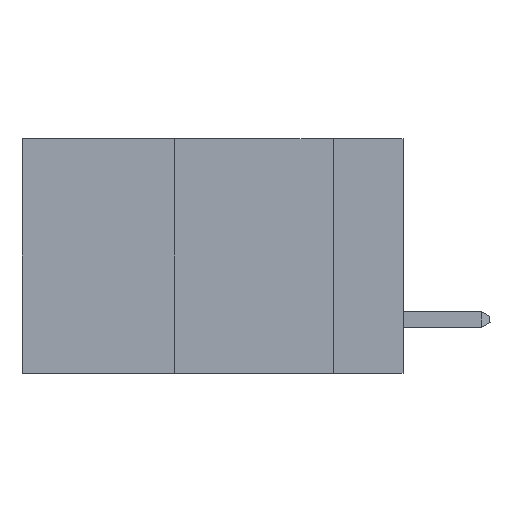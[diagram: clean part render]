
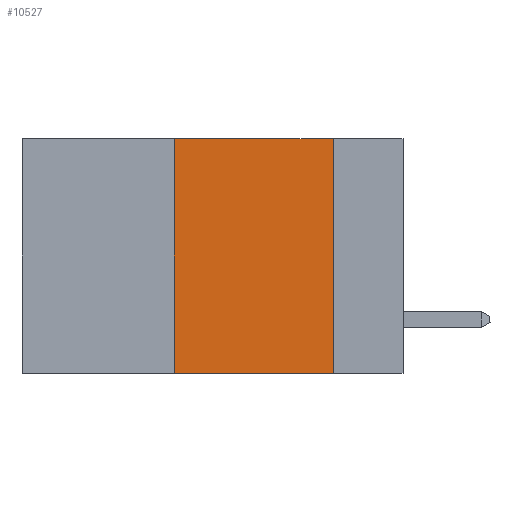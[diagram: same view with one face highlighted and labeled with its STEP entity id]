
A CAD part, left-side view. The second image highlights one B-rep face of the part: STEP entity #10527.
In plain terms, the highlighted planar face has unit normal (-1, 0, 0).
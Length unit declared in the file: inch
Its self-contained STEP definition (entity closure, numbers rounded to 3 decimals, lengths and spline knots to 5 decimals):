
#149 = VECTOR ( 'NONE', #7388, 39.37008 ) ;
#1104 = LINE ( 'NONE', #13494, #13376 ) ;
#1398 = CARTESIAN_POINT ( 'NONE',  ( 0., 0.6, 0. ) ) ;
#1529 = VERTEX_POINT ( 'NONE', #11540 ) ;
#1940 = PLANE ( 'NONE',  #2720 ) ;
#2425 = CARTESIAN_POINT ( 'NONE',  ( 0., 0.11, 0. ) ) ;
#2720 = AXIS2_PLACEMENT_3D ( 'NONE', #8182, #13185, #10703 ) ;
#2836 = FACE_OUTER_BOUND ( 'NONE', #13644, .T. ) ;
#3907 = ORIENTED_EDGE ( 'NONE', *, *, #10323, .F. ) ;
#4957 = VERTEX_POINT ( 'NONE', #9280 ) ;
#4985 = DIRECTION ( 'NONE',  ( 0., -1., 0. ) ) ;
#5191 = CARTESIAN_POINT ( 'NONE',  ( 0., 0.11, 0. ) ) ;
#5488 = ORIENTED_EDGE ( 'NONE', *, *, #15111, .F. ) ;
#6580 = LINE ( 'NONE', #1398, #9416 ) ;
#7388 = DIRECTION ( 'NONE',  ( 0., 0., -1. ) ) ;
#7775 = LINE ( 'NONE', #12483, #15484 ) ;
#7807 = VERTEX_POINT ( 'NONE', #13241 ) ;
#8182 = CARTESIAN_POINT ( 'NONE',  ( 0., 0.6, 0. ) ) ;
#9280 = CARTESIAN_POINT ( 'NONE',  ( 0., 0.36, 0. ) ) ;
#9416 = VECTOR ( 'NONE', #4985, 39.37008 ) ;
#9549 = VERTEX_POINT ( 'NONE', #5191 ) ;
#10323 = EDGE_CURVE ( 'NONE', #9549, #1529, #10918, .T. ) ;
#10340 = ORIENTED_EDGE ( 'NONE', *, *, #12864, .T. ) ;
#10527 = ADVANCED_FACE ( 'NONE', ( #2836 ), #1940, .F. ) ;
#10703 = DIRECTION ( 'NONE',  ( 0., 0., -1. ) ) ;
#10918 = LINE ( 'NONE', #2425, #149 ) ;
#11079 = ORIENTED_EDGE ( 'NONE', *, *, #13691, .F. ) ;
#11540 = CARTESIAN_POINT ( 'NONE',  ( 0., 0.11, -0.37 ) ) ;
#12483 = CARTESIAN_POINT ( 'NONE',  ( 0., 0.6, -0.37 ) ) ;
#12536 = DIRECTION ( 'NONE',  ( 0., -1., 0. ) ) ;
#12864 = EDGE_CURVE ( 'NONE', #7807, #1529, #7775, .T. ) ;
#13185 = DIRECTION ( 'NONE',  ( 1., 0., 0. ) ) ;
#13241 = CARTESIAN_POINT ( 'NONE',  ( 0., 0.36, -0.37 ) ) ;
#13336 = DIRECTION ( 'NONE',  ( 0., 0., 1. ) ) ;
#13376 = VECTOR ( 'NONE', #13336, 39.37008 ) ;
#13494 = CARTESIAN_POINT ( 'NONE',  ( 0., 0.36, 0. ) ) ;
#13644 = EDGE_LOOP ( 'NONE', ( #3907, #5488, #11079, #10340 ) ) ;
#13691 = EDGE_CURVE ( 'NONE', #7807, #4957, #1104, .T. ) ;
#15111 = EDGE_CURVE ( 'NONE', #4957, #9549, #6580, .T. ) ;
#15484 = VECTOR ( 'NONE', #12536, 39.37008 ) ;
